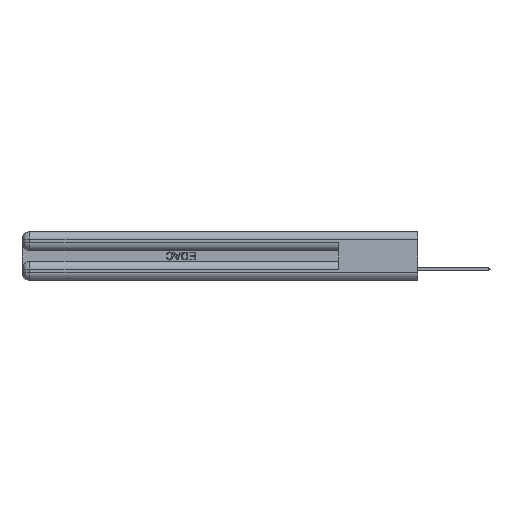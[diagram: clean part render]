
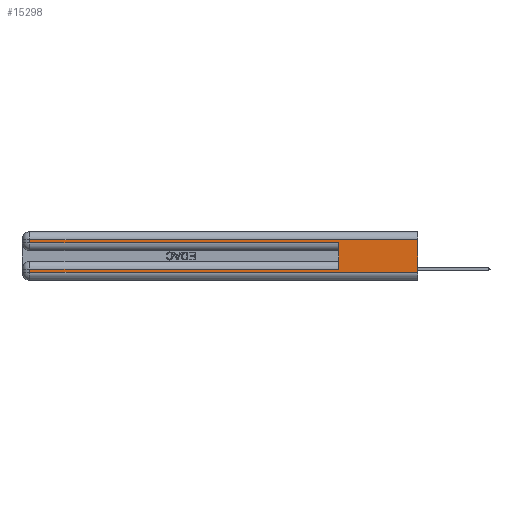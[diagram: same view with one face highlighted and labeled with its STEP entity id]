
A CAD part, left-side view. The second image highlights one B-rep face of the part: STEP entity #15298.
In plain terms, the highlighted planar face has unit normal (-1, 0, 0).
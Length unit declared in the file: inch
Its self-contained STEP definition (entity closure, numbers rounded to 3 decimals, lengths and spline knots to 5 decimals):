
#263 = EDGE_CURVE ( 'NONE', #1808, #45232, #22154, .T. ) ;
#1808 = VERTEX_POINT ( 'NONE', #27931 ) ;
#1947 = VECTOR ( 'NONE', #43618, 39.37008 ) ;
#2075 = EDGE_CURVE ( 'NONE', #25866, #17812, #38001, .T. ) ;
#3009 = LINE ( 'NONE', #6843, #10093 ) ;
#3914 = CARTESIAN_POINT ( 'NONE',  ( 0., 0.6, 0.285 ) ) ;
#4214 = VECTOR ( 'NONE', #48951, 39.37008 ) ;
#4579 = VECTOR ( 'NONE', #12992, 39.37008 ) ;
#5268 = PLANE ( 'NONE',  #5396 ) ;
#5396 = AXIS2_PLACEMENT_3D ( 'NONE', #41214, #31443, #27457 ) ;
#6672 = DIRECTION ( 'NONE',  ( 0., 0., -1. ) ) ;
#6843 = CARTESIAN_POINT ( 'NONE',  ( 0., 2.94, 0.37 ) ) ;
#7326 = CARTESIAN_POINT ( 'NONE',  ( 0., 0.6, 0.085 ) ) ;
#7327 = VERTEX_POINT ( 'NONE', #10677 ) ;
#8673 = VECTOR ( 'NONE', #40199, 39.37008 ) ;
#9268 = ORIENTED_EDGE ( 'NONE', *, *, #263, .T. ) ;
#9644 = DIRECTION ( 'NONE',  ( 0., 1., 0. ) ) ;
#10093 = VECTOR ( 'NONE', #6672, 39.37008 ) ;
#10561 = DIRECTION ( 'NONE',  ( 0., 0., -1. ) ) ;
#10677 = CARTESIAN_POINT ( 'NONE',  ( 0., 2.94, 0.085 ) ) ;
#10730 = EDGE_CURVE ( 'NONE', #38591, #7327, #40860, .T. ) ;
#12082 = CARTESIAN_POINT ( 'NONE',  ( 0., 0., 0.085 ) ) ;
#12777 = EDGE_CURVE ( 'NONE', #25866, #30514, #44285, .T. ) ;
#12992 = DIRECTION ( 'NONE',  ( 0., 0., 1. ) ) ;
#13741 = FACE_OUTER_BOUND ( 'NONE', #34325, .T. ) ;
#14270 = CARTESIAN_POINT ( 'NONE',  ( 0., 2.94, 0.31 ) ) ;
#14717 = VECTOR ( 'NONE', #38737, 39.37008 ) ;
#15298 = ADVANCED_FACE ( 'NONE', ( #13741 ), #5268, .F. ) ;
#15383 = ORIENTED_EDGE ( 'NONE', *, *, #15688, .T. ) ;
#15688 = EDGE_CURVE ( 'NONE', #17812, #1808, #3009, .T. ) ;
#16125 = ORIENTED_EDGE ( 'NONE', *, *, #12777, .F. ) ;
#16964 = EDGE_CURVE ( 'NONE', #38591, #45232, #45135, .T. ) ;
#17812 = VERTEX_POINT ( 'NONE', #14270 ) ;
#18676 = CARTESIAN_POINT ( 'NONE',  ( 0., 2.94, 0.37 ) ) ;
#18825 = LINE ( 'NONE', #20709, #8673 ) ;
#19802 = ORIENTED_EDGE ( 'NONE', *, *, #10730, .T. ) ;
#20047 = CARTESIAN_POINT ( 'NONE',  ( 0., 0., 0.06 ) ) ;
#20512 = ORIENTED_EDGE ( 'NONE', *, *, #24791, .T. ) ;
#20709 = CARTESIAN_POINT ( 'NONE',  ( 0., 0., 0.06 ) ) ;
#21881 = CARTESIAN_POINT ( 'NONE',  ( 0., 0., 0.37 ) ) ;
#22154 = LINE ( 'NONE', #35782, #1947 ) ;
#22412 = EDGE_CURVE ( 'NONE', #39755, #30514, #18825, .T. ) ;
#23952 = VECTOR ( 'NONE', #10561, 39.37008 ) ;
#24791 = EDGE_CURVE ( 'NONE', #7327, #39755, #43530, .T. ) ;
#25866 = VERTEX_POINT ( 'NONE', #43169 ) ;
#27457 = DIRECTION ( 'NONE',  ( 0., 0., -1. ) ) ;
#27806 = VECTOR ( 'NONE', #9644, 39.37008 ) ;
#27931 = CARTESIAN_POINT ( 'NONE',  ( 0., 2.94, 0.285 ) ) ;
#30514 = VERTEX_POINT ( 'NONE', #20047 ) ;
#31443 = DIRECTION ( 'NONE',  ( 1., 0., 0. ) ) ;
#33855 = CARTESIAN_POINT ( 'NONE',  ( 0., 2.94, 0.06 ) ) ;
#34325 = EDGE_LOOP ( 'NONE', ( #16125, #48901, #15383, #9268, #42166, #19802, #20512, #34381 ) ) ;
#34381 = ORIENTED_EDGE ( 'NONE', *, *, #22412, .T. ) ;
#34771 = CARTESIAN_POINT ( 'NONE',  ( 0., 0.6, 0.145 ) ) ;
#35782 = CARTESIAN_POINT ( 'NONE',  ( 0., 0., 0.285 ) ) ;
#38001 = LINE ( 'NONE', #39629, #27806 ) ;
#38591 = VERTEX_POINT ( 'NONE', #7326 ) ;
#38737 = DIRECTION ( 'NONE',  ( 0., 1., 0. ) ) ;
#39629 = CARTESIAN_POINT ( 'NONE',  ( 0., 0., 0.31 ) ) ;
#39755 = VERTEX_POINT ( 'NONE', #33855 ) ;
#40199 = DIRECTION ( 'NONE',  ( 0., -1., 0. ) ) ;
#40860 = LINE ( 'NONE', #12082, #14717 ) ;
#41214 = CARTESIAN_POINT ( 'NONE',  ( 0., 0., 0.37 ) ) ;
#42166 = ORIENTED_EDGE ( 'NONE', *, *, #16964, .F. ) ;
#43169 = CARTESIAN_POINT ( 'NONE',  ( 0., 0., 0.31 ) ) ;
#43530 = LINE ( 'NONE', #18676, #4214 ) ;
#43618 = DIRECTION ( 'NONE',  ( 0., -1., 0. ) ) ;
#44285 = LINE ( 'NONE', #21881, #23952 ) ;
#45135 = LINE ( 'NONE', #34771, #4579 ) ;
#45232 = VERTEX_POINT ( 'NONE', #3914 ) ;
#48901 = ORIENTED_EDGE ( 'NONE', *, *, #2075, .T. ) ;
#48951 = DIRECTION ( 'NONE',  ( 0., 0., -1. ) ) ;
